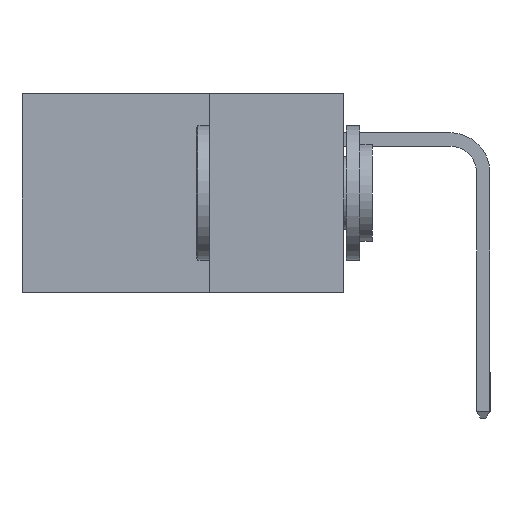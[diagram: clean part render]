
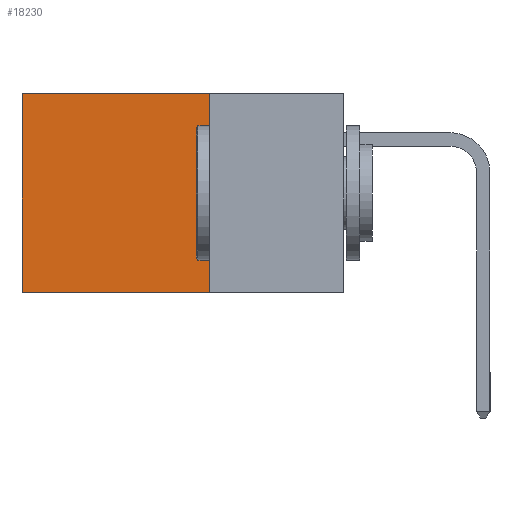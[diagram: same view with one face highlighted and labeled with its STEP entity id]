
A CAD part, left-side view. The second image highlights one B-rep face of the part: STEP entity #18230.
In plain terms, the highlighted planar face has unit normal (-1, 0, 0).
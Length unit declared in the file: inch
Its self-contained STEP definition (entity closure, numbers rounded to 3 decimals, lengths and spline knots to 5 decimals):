
#141 = VERTEX_POINT ( 'NONE', #8303 ) ;
#787 = DIRECTION ( 'NONE',  ( 1., 0., 0. ) ) ;
#1424 = CARTESIAN_POINT ( 'NONE',  ( 0.298, 0.6, 0. ) ) ;
#3901 = EDGE_CURVE ( 'NONE', #141, #7010, #11549, .T. ) ;
#4765 = FACE_OUTER_BOUND ( 'NONE', #14217, .T. ) ;
#5434 = LINE ( 'NONE', #16076, #16581 ) ;
#6167 = LINE ( 'NONE', #12533, #7593 ) ;
#6995 = DIRECTION ( 'NONE',  ( 0., 1., 0. ) ) ;
#7010 = VERTEX_POINT ( 'NONE', #1424 ) ;
#7348 = EDGE_CURVE ( 'NONE', #141, #15990, #6167, .T. ) ;
#7593 = VECTOR ( 'NONE', #18679, 39.37008 ) ;
#8303 = CARTESIAN_POINT ( 'NONE',  ( 0.298, 0.25, 0. ) ) ;
#8416 = PLANE ( 'NONE',  #14535 ) ;
#8685 = CARTESIAN_POINT ( 'NONE',  ( 0.298, 0.25, -0.37 ) ) ;
#8705 = DIRECTION ( 'NONE',  ( 0., 0., -1. ) ) ;
#9240 = ORIENTED_EDGE ( 'NONE', *, *, #14743, .F. ) ;
#9879 = CARTESIAN_POINT ( 'NONE',  ( 0.298, 0.25, 0. ) ) ;
#10442 = CARTESIAN_POINT ( 'NONE',  ( 0.298, 0.25, 0. ) ) ;
#10552 = VECTOR ( 'NONE', #8705, 39.37008 ) ;
#11380 = EDGE_CURVE ( 'NONE', #7010, #18576, #19343, .T. ) ;
#11416 = DIRECTION ( 'NONE',  ( 0., 0., -1. ) ) ;
#11549 = LINE ( 'NONE', #10442, #19625 ) ;
#12533 = CARTESIAN_POINT ( 'NONE',  ( 0.298, 0.25, 0. ) ) ;
#13160 = DIRECTION ( 'NONE',  ( 0., 1., 0. ) ) ;
#13246 = ORIENTED_EDGE ( 'NONE', *, *, #7348, .F. ) ;
#14007 = ORIENTED_EDGE ( 'NONE', *, *, #11380, .T. ) ;
#14217 = EDGE_LOOP ( 'NONE', ( #14007, #9240, #13246, #18944 ) ) ;
#14535 = AXIS2_PLACEMENT_3D ( 'NONE', #9879, #787, #11416 ) ;
#14743 = EDGE_CURVE ( 'NONE', #15990, #18576, #5434, .T. ) ;
#15990 = VERTEX_POINT ( 'NONE', #8685 ) ;
#16076 = CARTESIAN_POINT ( 'NONE',  ( 0.298, 0.25, -0.37 ) ) ;
#16520 = CARTESIAN_POINT ( 'NONE',  ( 0.298, 0.6, -0.37 ) ) ;
#16581 = VECTOR ( 'NONE', #6995, 39.37008 ) ;
#18230 = ADVANCED_FACE ( 'NONE', ( #4765 ), #8416, .F. ) ;
#18576 = VERTEX_POINT ( 'NONE', #16520 ) ;
#18679 = DIRECTION ( 'NONE',  ( 0., 0., -1. ) ) ;
#18944 = ORIENTED_EDGE ( 'NONE', *, *, #3901, .T. ) ;
#19200 = CARTESIAN_POINT ( 'NONE',  ( 0.298, 0.6, 0. ) ) ;
#19343 = LINE ( 'NONE', #19200, #10552 ) ;
#19625 = VECTOR ( 'NONE', #13160, 39.37008 ) ;
